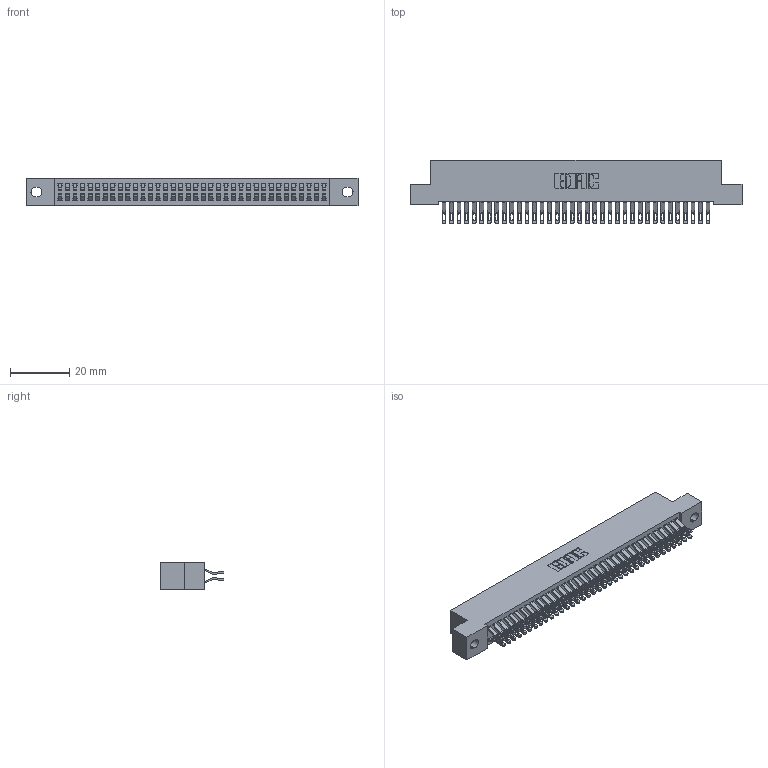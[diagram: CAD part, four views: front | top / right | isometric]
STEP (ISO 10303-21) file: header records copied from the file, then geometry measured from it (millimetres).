
FILE_DESCRIPTION (( 'STEP AP203' ), '1' );
FILE_NAME ('392-072-555-202.STEP', '2018-08-18T00:15:46', ( '' ), ( '' ), 'SwSTEP 2.0', 'SolidWorks 2016', '' );
FILE_SCHEMA (( 'CONFIG_CONTROL_DESIGN' ));
Length unit declared in the file: inch
Products named in the file (3): 342 Part_.128 Slot; 345-292-001_555 Tail; 392-072-555-202
Assembly tree (73 placements, depth 2):
  392-072-555-202
    342 Part_.128 Slot
    345-292-001_555 Tail  x72
Bounding box: 111.76 x 21.47 x 9.4 mm (x, y, z)
Volume: 10161.2 mm3; surface area: 16848.1 mm2
Topology: 73 solids, 73 shells, 4290 faces, 13487 edges, 8990 vertices
Faces by surface type: plane 2518, cylinder 1772
Entity records: 24265 total; most frequent: CARTESIAN_POINT 4064, ORIENTED_EDGE 3970, DIRECTION 3453, EDGE_CURVE 1985, LINE 1837, VECTOR 1837, VERTEX_POINT 1322, AXIS2_PLACEMENT_3D 808
